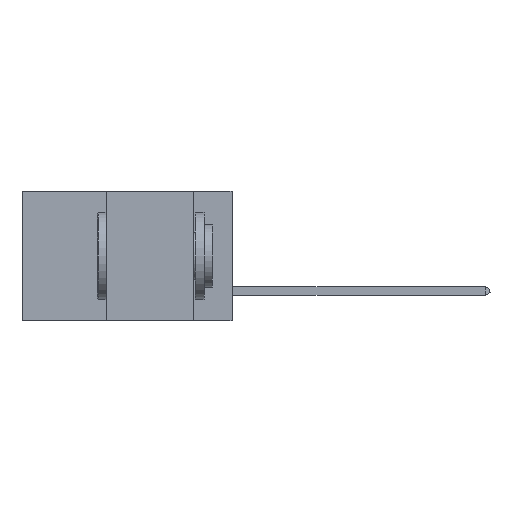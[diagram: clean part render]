
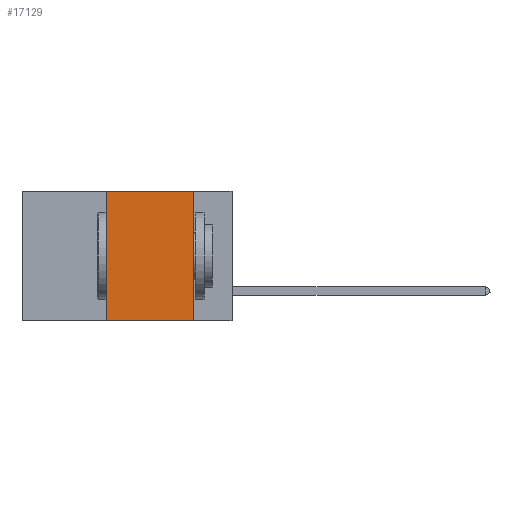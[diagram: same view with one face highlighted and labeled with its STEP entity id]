
A CAD part, left-side view. The second image highlights one B-rep face of the part: STEP entity #17129.
In plain terms, the highlighted planar face has unit normal (-1, 0, 0).
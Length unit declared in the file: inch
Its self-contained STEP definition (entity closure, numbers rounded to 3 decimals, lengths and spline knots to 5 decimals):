
#409 = LINE ( 'NONE', #2520, #5320 ) ;
#564 = VECTOR ( 'NONE', #15753, 39.37008 ) ;
#2520 = CARTESIAN_POINT ( 'NONE',  ( 0., 0.36, 0. ) ) ;
#3269 = VERTEX_POINT ( 'NONE', #22940 ) ;
#3276 = VERTEX_POINT ( 'NONE', #15550 ) ;
#3803 = LINE ( 'NONE', #28502, #27187 ) ;
#3875 = LINE ( 'NONE', #28597, #26908 ) ;
#4172 = AXIS2_PLACEMENT_3D ( 'NONE', #4226, #17408, #22046 ) ;
#4226 = CARTESIAN_POINT ( 'NONE',  ( 0., 0.6, 0. ) ) ;
#5320 = VECTOR ( 'NONE', #9138, 39.37008 ) ;
#6104 = VERTEX_POINT ( 'NONE', #27236 ) ;
#6425 = EDGE_CURVE ( 'NONE', #6104, #3269, #3803, .T. ) ;
#8872 = VERTEX_POINT ( 'NONE', #25333 ) ;
#9138 = DIRECTION ( 'NONE',  ( 0., 0., 1. ) ) ;
#10734 = PLANE ( 'NONE',  #4172 ) ;
#10754 = EDGE_CURVE ( 'NONE', #8872, #6104, #409, .T. ) ;
#11033 = ORIENTED_EDGE ( 'NONE', *, *, #20067, .T. ) ;
#13290 = LINE ( 'NONE', #20094, #564 ) ;
#14369 = ORIENTED_EDGE ( 'NONE', *, *, #6425, .F. ) ;
#14938 = DIRECTION ( 'NONE',  ( 0., -1., 0. ) ) ;
#15338 = DIRECTION ( 'NONE',  ( 0., 0., -1. ) ) ;
#15550 = CARTESIAN_POINT ( 'NONE',  ( 0., 0.11, -0.37 ) ) ;
#15753 = DIRECTION ( 'NONE',  ( 0., -1., 0. ) ) ;
#16663 = EDGE_LOOP ( 'NONE', ( #26925, #14369, #27817, #11033 ) ) ;
#17129 = ADVANCED_FACE ( 'NONE', ( #22233 ), #10734, .F. ) ;
#17408 = DIRECTION ( 'NONE',  ( 1., 0., 0. ) ) ;
#20067 = EDGE_CURVE ( 'NONE', #8872, #3276, #13290, .T. ) ;
#20094 = CARTESIAN_POINT ( 'NONE',  ( 0., 0.6, -0.37 ) ) ;
#22046 = DIRECTION ( 'NONE',  ( 0., 0., -1. ) ) ;
#22233 = FACE_OUTER_BOUND ( 'NONE', #16663, .T. ) ;
#22940 = CARTESIAN_POINT ( 'NONE',  ( 0., 0.11, 0. ) ) ;
#23300 = EDGE_CURVE ( 'NONE', #3269, #3276, #3875, .T. ) ;
#25333 = CARTESIAN_POINT ( 'NONE',  ( 0., 0.36, -0.37 ) ) ;
#26908 = VECTOR ( 'NONE', #15338, 39.37008 ) ;
#26925 = ORIENTED_EDGE ( 'NONE', *, *, #23300, .F. ) ;
#27187 = VECTOR ( 'NONE', #14938, 39.37008 ) ;
#27236 = CARTESIAN_POINT ( 'NONE',  ( 0., 0.36, 0. ) ) ;
#27817 = ORIENTED_EDGE ( 'NONE', *, *, #10754, .F. ) ;
#28502 = CARTESIAN_POINT ( 'NONE',  ( 0., 0.6, 0. ) ) ;
#28597 = CARTESIAN_POINT ( 'NONE',  ( 0., 0.11, 0. ) ) ;
